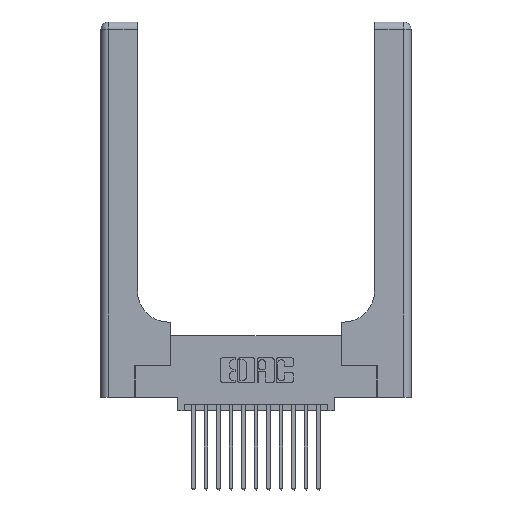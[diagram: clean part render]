
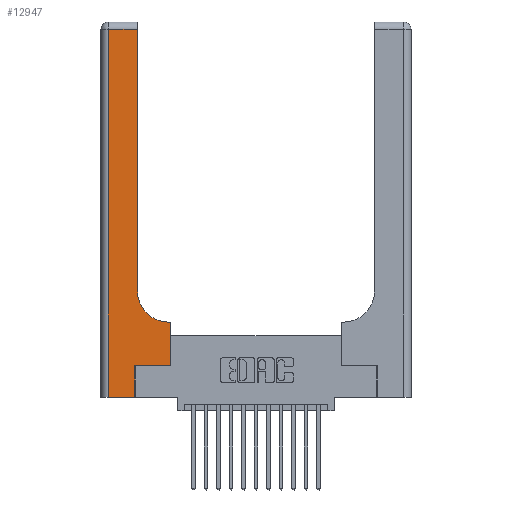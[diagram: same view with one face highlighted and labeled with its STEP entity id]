
A CAD part, top view. The second image highlights one B-rep face of the part: STEP entity #12947.
In plain terms, the highlighted planar face has unit normal (0, 0, 1).
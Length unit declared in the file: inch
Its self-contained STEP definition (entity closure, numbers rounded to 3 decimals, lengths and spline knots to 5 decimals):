
#323 = EDGE_LOOP ( 'NONE', ( #3946, #4402, #11828, #15907, #1450, #12697, #1906, #13124, #2362 ) ) ;
#1151 = EDGE_CURVE ( 'NONE', #4782, #15149, #13393, .T. ) ;
#1245 = LINE ( 'NONE', #4395, #15724 ) ;
#1450 = ORIENTED_EDGE ( 'NONE', *, *, #8209, .T. ) ;
#1492 = CARTESIAN_POINT ( 'NONE',  ( 0.06, 3., 0.37 ) ) ;
#1718 = DIRECTION ( 'NONE',  ( 0., 0., -1. ) ) ;
#1906 = ORIENTED_EDGE ( 'NONE', *, *, #14374, .T. ) ;
#1976 = CIRCLE ( 'NONE', #11703, 0.25 ) ;
#2362 = ORIENTED_EDGE ( 'NONE', *, *, #13932, .T. ) ;
#2934 = DIRECTION ( 'NONE',  ( 0., -1., 0. ) ) ;
#3343 = LINE ( 'NONE', #1492, #6713 ) ;
#3946 = ORIENTED_EDGE ( 'NONE', *, *, #4382, .T. ) ;
#4382 = EDGE_CURVE ( 'NONE', #12396, #4782, #5938, .T. ) ;
#4395 = CARTESIAN_POINT ( 'NONE',  ( 0.269, 0., 0.37 ) ) ;
#4402 = ORIENTED_EDGE ( 'NONE', *, *, #1151, .T. ) ;
#4507 = VERTEX_POINT ( 'NONE', #17631 ) ;
#4533 = VERTEX_POINT ( 'NONE', #6708 ) ;
#4782 = VERTEX_POINT ( 'NONE', #14378 ) ;
#5176 = EDGE_CURVE ( 'NONE', #11717, #4533, #7421, .T. ) ;
#5938 = LINE ( 'NONE', #13302, #12887 ) ;
#6065 = CARTESIAN_POINT ( 'NONE',  ( 0.06, 0., 0.37 ) ) ;
#6224 = LINE ( 'NONE', #8248, #12735 ) ;
#6288 = DIRECTION ( 'NONE',  ( 0., 0., -1. ) ) ;
#6468 = VECTOR ( 'NONE', #15236, 39.37008 ) ;
#6708 = CARTESIAN_POINT ( 'NONE',  ( 0.269, 0., 0.37 ) ) ;
#6713 = VECTOR ( 'NONE', #2934, 39.37008 ) ;
#6946 = VERTEX_POINT ( 'NONE', #11212 ) ;
#7421 = LINE ( 'NONE', #17858, #14326 ) ;
#7641 = PLANE ( 'NONE',  #9021 ) ;
#8026 = VERTEX_POINT ( 'NONE', #17624 ) ;
#8209 = EDGE_CURVE ( 'NONE', #4533, #6946, #1245, .T. ) ;
#8248 = CARTESIAN_POINT ( 'NONE',  ( 0.5585, 0.25, 0.37 ) ) ;
#8555 = LINE ( 'NONE', #12686, #11796 ) ;
#8906 = CARTESIAN_POINT ( 'NONE',  ( 0.5585, 0.25, 0.37 ) ) ;
#9021 = AXIS2_PLACEMENT_3D ( 'NONE', #14566, #6288, #15949 ) ;
#9184 = CARTESIAN_POINT ( 'NONE',  ( 0.2915, 0.6, 0.37 ) ) ;
#9549 = FACE_OUTER_BOUND ( 'NONE', #323, .T. ) ;
#9634 = DIRECTION ( 'NONE',  ( 0., 1., 0. ) ) ;
#9869 = EDGE_CURVE ( 'NONE', #6946, #15692, #8555, .T. ) ;
#9878 = LINE ( 'NONE', #9184, #13559 ) ;
#10173 = CARTESIAN_POINT ( 'NONE',  ( 0.5415, 0.85, 0.37 ) ) ;
#10330 = CARTESIAN_POINT ( 'NONE',  ( 0.2915, 0.85, 0.37 ) ) ;
#10553 = DIRECTION ( 'NONE',  ( -1., 0., 0. ) ) ;
#11212 = CARTESIAN_POINT ( 'NONE',  ( 0.269, 0.25, 0.37 ) ) ;
#11582 = DIRECTION ( 'NONE',  ( 1., 0., 0. ) ) ;
#11608 = CARTESIAN_POINT ( 'NONE',  ( 0.06, 2.94, 0.37 ) ) ;
#11703 = AXIS2_PLACEMENT_3D ( 'NONE', #10173, #1718, #11582 ) ;
#11717 = VERTEX_POINT ( 'NONE', #6065 ) ;
#11796 = VECTOR ( 'NONE', #14067, 39.37008 ) ;
#11828 = ORIENTED_EDGE ( 'NONE', *, *, #13369, .T. ) ;
#12388 = DIRECTION ( 'NONE',  ( 1., 0., 0. ) ) ;
#12396 = VERTEX_POINT ( 'NONE', #10330 ) ;
#12686 = CARTESIAN_POINT ( 'NONE',  ( 0.269, 0.25, 0.37 ) ) ;
#12697 = ORIENTED_EDGE ( 'NONE', *, *, #9869, .T. ) ;
#12735 = VECTOR ( 'NONE', #9634, 39.37008 ) ;
#12887 = VECTOR ( 'NONE', #14681, 39.37008 ) ;
#12947 = ADVANCED_FACE ( 'NONE', ( #9549 ), #7641, .F. ) ;
#13124 = ORIENTED_EDGE ( 'NONE', *, *, #15209, .T. ) ;
#13302 = CARTESIAN_POINT ( 'NONE',  ( 0.2915, 3., 0.37 ) ) ;
#13369 = EDGE_CURVE ( 'NONE', #15149, #11717, #3343, .T. ) ;
#13393 = LINE ( 'NONE', #14055, #6468 ) ;
#13559 = VECTOR ( 'NONE', #10553, 39.37008 ) ;
#13932 = EDGE_CURVE ( 'NONE', #8026, #12396, #1976, .T. ) ;
#14055 = CARTESIAN_POINT ( 'NONE',  ( 0., 2.94, 0.37 ) ) ;
#14067 = DIRECTION ( 'NONE',  ( 1., 0., 0. ) ) ;
#14326 = VECTOR ( 'NONE', #12388, 39.37008 ) ;
#14374 = EDGE_CURVE ( 'NONE', #15692, #4507, #6224, .T. ) ;
#14378 = CARTESIAN_POINT ( 'NONE',  ( 0.2915, 2.94, 0.37 ) ) ;
#14566 = CARTESIAN_POINT ( 'NONE',  ( 0., 3., 0.37 ) ) ;
#14681 = DIRECTION ( 'NONE',  ( 0., 1., 0. ) ) ;
#15149 = VERTEX_POINT ( 'NONE', #11608 ) ;
#15209 = EDGE_CURVE ( 'NONE', #4507, #8026, #9878, .T. ) ;
#15236 = DIRECTION ( 'NONE',  ( -1., 0., 0. ) ) ;
#15692 = VERTEX_POINT ( 'NONE', #8906 ) ;
#15724 = VECTOR ( 'NONE', #16853, 39.37008 ) ;
#15907 = ORIENTED_EDGE ( 'NONE', *, *, #5176, .T. ) ;
#15949 = DIRECTION ( 'NONE',  ( -1., 0., 0. ) ) ;
#16853 = DIRECTION ( 'NONE',  ( 0., 1., 0. ) ) ;
#17624 = CARTESIAN_POINT ( 'NONE',  ( 0.5415, 0.6, 0.37 ) ) ;
#17631 = CARTESIAN_POINT ( 'NONE',  ( 0.5585, 0.6, 0.37 ) ) ;
#17858 = CARTESIAN_POINT ( 'NONE',  ( 0., 0., 0.37 ) ) ;
